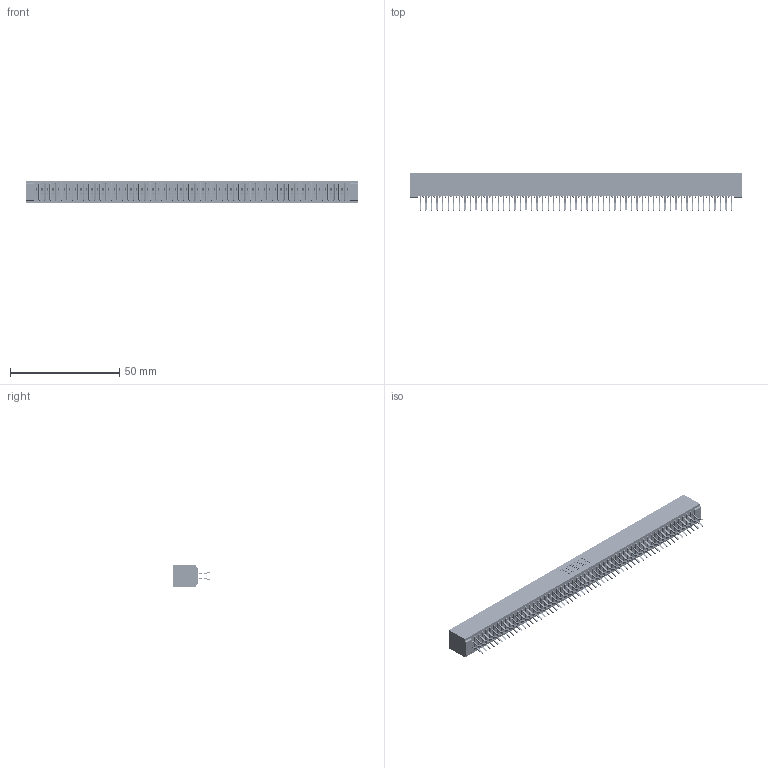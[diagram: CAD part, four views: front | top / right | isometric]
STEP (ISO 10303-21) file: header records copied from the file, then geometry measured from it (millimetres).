
FILE_DESCRIPTION (( 'STEP AP203' ), '1' );
FILE_NAME ('391-114-556-201.STEP', '2018-08-09T22:51:11', ( '' ), ( '' ), 'SwSTEP 2.0', 'SolidWorks 2016', '' );
FILE_SCHEMA (( 'CONFIG_CONTROL_DESIGN' ));
Length unit declared in the file: inch
Products named in the file (3): 341 Part_No Mounting Lugs; 341-292-001_341-292-156; 391-114-556-201
Assembly tree (115 placements, depth 2):
  391-114-556-201
    341 Part_No Mounting Lugs
    341-292-001_341-292-156  x114
Bounding box: 151.76 x 17.07 x 10.16 mm (x, y, z)
Volume: 852.1 mm3; surface area: 21807.1 mm2
Topology: 114 solids, 115 shells, 8086 faces, 23491 edges, 15238 vertices
Faces by surface type: plane 4622, cylinder 3236, sphere 116, torus 112
Entity records: 66846 total; most frequent: CARTESIAN_POINT 11111, ORIENTED_EDGE 11042, DIRECTION 10775, EDGE_CURVE 5521, VECTOR 4475, LINE 4475, VERTEX_POINT 3486, AXIS2_PLACEMENT_3D 3150
